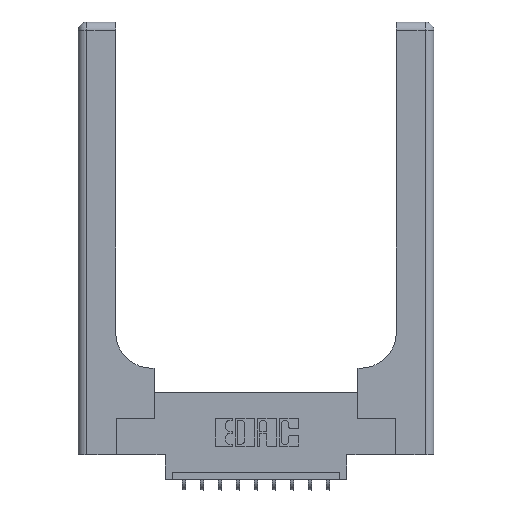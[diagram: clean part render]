
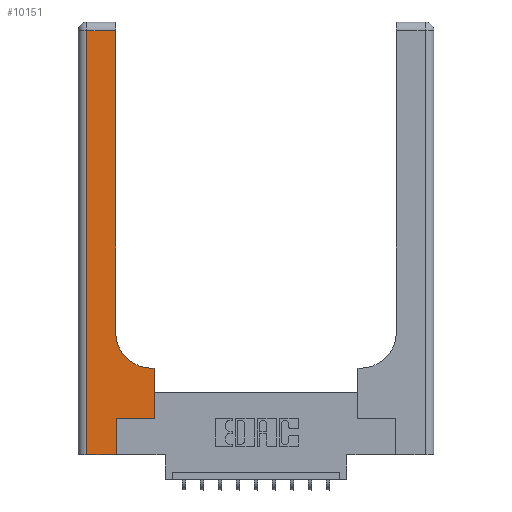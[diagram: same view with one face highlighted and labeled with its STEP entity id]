
A CAD part, top view. The second image highlights one B-rep face of the part: STEP entity #10151.
In plain terms, the highlighted planar face has unit normal (0, 0, 1).
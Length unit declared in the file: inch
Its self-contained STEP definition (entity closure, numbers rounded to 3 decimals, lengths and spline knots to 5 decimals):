
#75 = ORIENTED_EDGE ( 'NONE', *, *, #2047, .T. ) ;
#223 = ORIENTED_EDGE ( 'NONE', *, *, #3643, .T. ) ;
#456 = EDGE_CURVE ( 'NONE', #11631, #4204, #10223, .T. ) ;
#457 = CARTESIAN_POINT ( 'NONE',  ( 0.528, 0.6, 0.37 ) ) ;
#540 = EDGE_CURVE ( 'NONE', #1558, #4107, #15469, .T. ) ;
#807 = CARTESIAN_POINT ( 'NONE',  ( 0.26, 0.85, 0.37 ) ) ;
#1131 = LINE ( 'NONE', #15837, #5339 ) ;
#1172 = CARTESIAN_POINT ( 'NONE',  ( 0.265, 0., 0.37 ) ) ;
#1558 = VERTEX_POINT ( 'NONE', #11366 ) ;
#2047 = EDGE_CURVE ( 'NONE', #9866, #8324, #4757, .T. ) ;
#2156 = CARTESIAN_POINT ( 'NONE',  ( 0.528, 0.25, 0.37 ) ) ;
#2348 = DIRECTION ( 'NONE',  ( 1., 0., 0. ) ) ;
#2504 = EDGE_LOOP ( 'NONE', ( #12700, #223, #6856, #3194, #15031, #75, #9986, #9460, #10900 ) ) ;
#2856 = DIRECTION ( 'NONE',  ( 0., 1., 0. ) ) ;
#3194 = ORIENTED_EDGE ( 'NONE', *, *, #5446, .T. ) ;
#3321 = VERTEX_POINT ( 'NONE', #1172 ) ;
#3428 = PLANE ( 'NONE',  #7322 ) ;
#3579 = VECTOR ( 'NONE', #13158, 39.37008 ) ;
#3643 = EDGE_CURVE ( 'NONE', #4204, #1558, #1131, .T. ) ;
#3879 = LINE ( 'NONE', #7364, #4940 ) ;
#4091 = DIRECTION ( 'NONE',  ( 1., 0., 0. ) ) ;
#4107 = VERTEX_POINT ( 'NONE', #11191 ) ;
#4204 = VERTEX_POINT ( 'NONE', #15043 ) ;
#4757 = LINE ( 'NONE', #8332, #11899 ) ;
#4895 = VECTOR ( 'NONE', #4091, 39.37008 ) ;
#4940 = VECTOR ( 'NONE', #6396, 39.37008 ) ;
#5217 = VECTOR ( 'NONE', #6756, 39.37008 ) ;
#5242 = EDGE_CURVE ( 'NONE', #15050, #8137, #13475, .T. ) ;
#5339 = VECTOR ( 'NONE', #6216, 39.37008 ) ;
#5446 = EDGE_CURVE ( 'NONE', #4107, #3321, #7823, .T. ) ;
#5609 = EDGE_CURVE ( 'NONE', #8324, #15050, #13199, .T. ) ;
#5882 = CARTESIAN_POINT ( 'NONE',  ( 0., 3., 0.37 ) ) ;
#6216 = DIRECTION ( 'NONE',  ( -1., 0., 0. ) ) ;
#6396 = DIRECTION ( 'NONE',  ( 0., 1., 0. ) ) ;
#6756 = DIRECTION ( 'NONE',  ( 0., 1., 0. ) ) ;
#6856 = ORIENTED_EDGE ( 'NONE', *, *, #540, .T. ) ;
#7046 = CARTESIAN_POINT ( 'NONE',  ( 0.51, 0.6, 0.37 ) ) ;
#7297 = AXIS2_PLACEMENT_3D ( 'NONE', #10747, #9380, #15604 ) ;
#7322 = AXIS2_PLACEMENT_3D ( 'NONE', #5882, #9600, #15361 ) ;
#7344 = CARTESIAN_POINT ( 'NONE',  ( 0.265, 0.25, 0.37 ) ) ;
#7364 = CARTESIAN_POINT ( 'NONE',  ( 0.265, 0., 0.37 ) ) ;
#7823 = LINE ( 'NONE', #9042, #4895 ) ;
#8137 = VERTEX_POINT ( 'NONE', #7046 ) ;
#8202 = DIRECTION ( 'NONE',  ( 0., -1., 0. ) ) ;
#8324 = VERTEX_POINT ( 'NONE', #8326 ) ;
#8326 = CARTESIAN_POINT ( 'NONE',  ( 0.528, 0.25, 0.37 ) ) ;
#8332 = CARTESIAN_POINT ( 'NONE',  ( 0.265, 0.25, 0.37 ) ) ;
#9042 = CARTESIAN_POINT ( 'NONE',  ( 0., 0., 0.37 ) ) ;
#9282 = FACE_OUTER_BOUND ( 'NONE', #2504, .T. ) ;
#9372 = EDGE_CURVE ( 'NONE', #3321, #9866, #3879, .T. ) ;
#9380 = DIRECTION ( 'NONE',  ( 0., 0., -1. ) ) ;
#9460 = ORIENTED_EDGE ( 'NONE', *, *, #5242, .T. ) ;
#9600 = DIRECTION ( 'NONE',  ( 0., 0., -1. ) ) ;
#9603 = EDGE_CURVE ( 'NONE', #8137, #11631, #14739, .T. ) ;
#9785 = CARTESIAN_POINT ( 'NONE',  ( 0.26, 0.6, 0.37 ) ) ;
#9866 = VERTEX_POINT ( 'NONE', #7344 ) ;
#9986 = ORIENTED_EDGE ( 'NONE', *, *, #5609, .T. ) ;
#10151 = ADVANCED_FACE ( 'NONE', ( #9282 ), #3428, .F. ) ;
#10223 = LINE ( 'NONE', #13913, #15386 ) ;
#10747 = CARTESIAN_POINT ( 'NONE',  ( 0.51, 0.85, 0.37 ) ) ;
#10900 = ORIENTED_EDGE ( 'NONE', *, *, #9603, .T. ) ;
#11191 = CARTESIAN_POINT ( 'NONE',  ( 0.06, 0., 0.37 ) ) ;
#11366 = CARTESIAN_POINT ( 'NONE',  ( 0.06, 2.94, 0.37 ) ) ;
#11631 = VERTEX_POINT ( 'NONE', #807 ) ;
#11899 = VECTOR ( 'NONE', #2348, 39.37008 ) ;
#12700 = ORIENTED_EDGE ( 'NONE', *, *, #456, .T. ) ;
#13158 = DIRECTION ( 'NONE',  ( -1., 0., 0. ) ) ;
#13199 = LINE ( 'NONE', #2156, #5217 ) ;
#13475 = LINE ( 'NONE', #9785, #3579 ) ;
#13913 = CARTESIAN_POINT ( 'NONE',  ( 0.26, 3., 0.37 ) ) ;
#14146 = CARTESIAN_POINT ( 'NONE',  ( 0.06, 3., 0.37 ) ) ;
#14602 = VECTOR ( 'NONE', #8202, 39.37008 ) ;
#14739 = CIRCLE ( 'NONE', #7297, 0.25 ) ;
#15031 = ORIENTED_EDGE ( 'NONE', *, *, #9372, .T. ) ;
#15043 = CARTESIAN_POINT ( 'NONE',  ( 0.26, 2.94, 0.37 ) ) ;
#15050 = VERTEX_POINT ( 'NONE', #457 ) ;
#15361 = DIRECTION ( 'NONE',  ( -1., 0., 0. ) ) ;
#15386 = VECTOR ( 'NONE', #2856, 39.37008 ) ;
#15469 = LINE ( 'NONE', #14146, #14602 ) ;
#15604 = DIRECTION ( 'NONE',  ( 1., 0., 0. ) ) ;
#15837 = CARTESIAN_POINT ( 'NONE',  ( 0., 2.94, 0.37 ) ) ;
